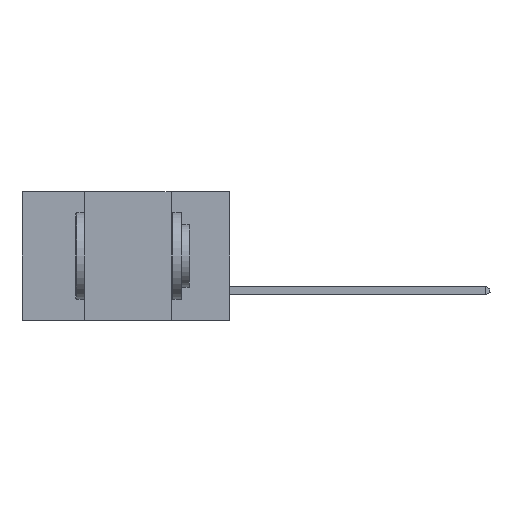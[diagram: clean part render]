
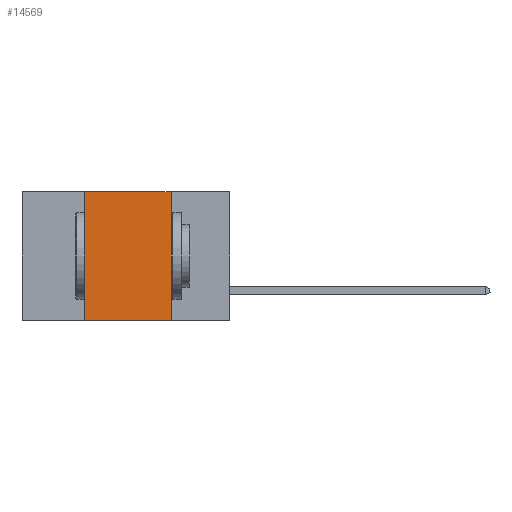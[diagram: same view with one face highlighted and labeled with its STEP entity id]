
A CAD part, left-side view. The second image highlights one B-rep face of the part: STEP entity #14569.
In plain terms, the highlighted planar face has unit normal (-1, 0, 0).
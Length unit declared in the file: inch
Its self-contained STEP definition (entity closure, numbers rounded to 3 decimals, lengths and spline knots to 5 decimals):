
#58 = EDGE_LOOP ( 'NONE', ( #16702, #17020, #5081, #17672 ) ) ;
#582 = DIRECTION ( 'NONE',  ( 0., 0., -1. ) ) ;
#2414 = VERTEX_POINT ( 'NONE', #14239 ) ;
#2425 = CARTESIAN_POINT ( 'NONE',  ( 0., 0.6, 0. ) ) ;
#2862 = DIRECTION ( 'NONE',  ( 1., 0., 0. ) ) ;
#4061 = LINE ( 'NONE', #12205, #11096 ) ;
#4486 = VECTOR ( 'NONE', #14693, 39.37008 ) ;
#4528 = DIRECTION ( 'NONE',  ( 0., 0., -1. ) ) ;
#5081 = ORIENTED_EDGE ( 'NONE', *, *, #7344, .F. ) ;
#5808 = DIRECTION ( 'NONE',  ( 0., 0., 1. ) ) ;
#6276 = CARTESIAN_POINT ( 'NONE',  ( 0., 0.6, 0. ) ) ;
#6980 = VECTOR ( 'NONE', #20709, 39.37008 ) ;
#7344 = EDGE_CURVE ( 'NONE', #13856, #17292, #11820, .T. ) ;
#7369 = LINE ( 'NONE', #7906, #4486 ) ;
#7906 = CARTESIAN_POINT ( 'NONE',  ( 0., 0.6, -0.37 ) ) ;
#8027 = VERTEX_POINT ( 'NONE', #10999 ) ;
#8078 = AXIS2_PLACEMENT_3D ( 'NONE', #6276, #2862, #4528 ) ;
#8383 = VECTOR ( 'NONE', #5808, 39.37008 ) ;
#9063 = EDGE_CURVE ( 'NONE', #17292, #8027, #14291, .T. ) ;
#9336 = CARTESIAN_POINT ( 'NONE',  ( 0., 0.42, 0. ) ) ;
#9519 = PLANE ( 'NONE',  #8078 ) ;
#10999 = CARTESIAN_POINT ( 'NONE',  ( 0., 0.17, 0. ) ) ;
#11096 = VECTOR ( 'NONE', #582, 39.37008 ) ;
#11206 = CARTESIAN_POINT ( 'NONE',  ( 0., 0.42, -0.37 ) ) ;
#11712 = CARTESIAN_POINT ( 'NONE',  ( 0., 0.42, 0. ) ) ;
#11820 = LINE ( 'NONE', #9336, #8383 ) ;
#12205 = CARTESIAN_POINT ( 'NONE',  ( 0., 0.17, 0. ) ) ;
#13856 = VERTEX_POINT ( 'NONE', #11206 ) ;
#14239 = CARTESIAN_POINT ( 'NONE',  ( 0., 0.17, -0.37 ) ) ;
#14291 = LINE ( 'NONE', #2425, #6980 ) ;
#14569 = ADVANCED_FACE ( 'NONE', ( #19791 ), #9519, .F. ) ;
#14693 = DIRECTION ( 'NONE',  ( 0., -1., 0. ) ) ;
#16702 = ORIENTED_EDGE ( 'NONE', *, *, #19016, .F. ) ;
#17020 = ORIENTED_EDGE ( 'NONE', *, *, #9063, .F. ) ;
#17292 = VERTEX_POINT ( 'NONE', #11712 ) ;
#17672 = ORIENTED_EDGE ( 'NONE', *, *, #21290, .T. ) ;
#19016 = EDGE_CURVE ( 'NONE', #8027, #2414, #4061, .T. ) ;
#19791 = FACE_OUTER_BOUND ( 'NONE', #58, .T. ) ;
#20709 = DIRECTION ( 'NONE',  ( 0., -1., 0. ) ) ;
#21290 = EDGE_CURVE ( 'NONE', #13856, #2414, #7369, .T. ) ;
